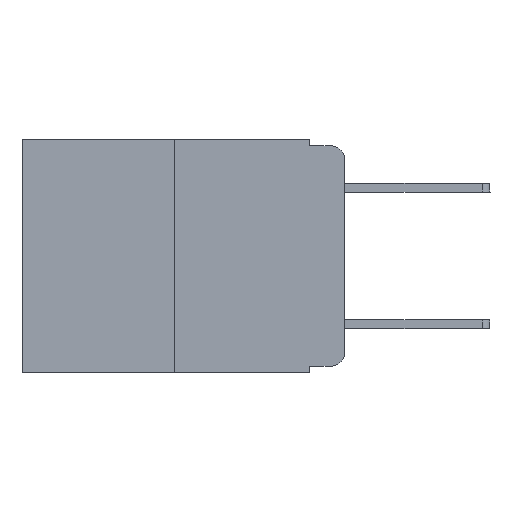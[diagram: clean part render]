
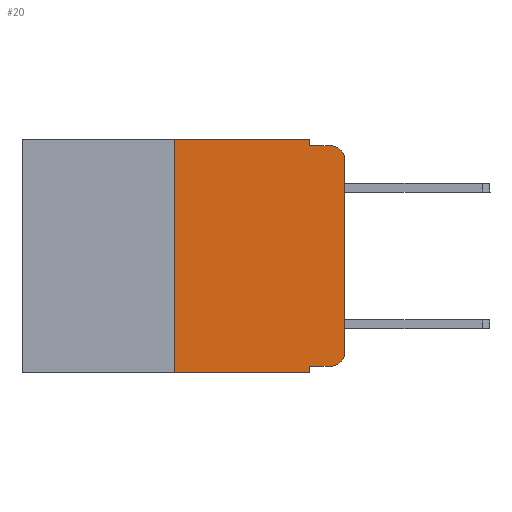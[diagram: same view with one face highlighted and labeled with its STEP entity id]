
A CAD part, left-side view. The second image highlights one B-rep face of the part: STEP entity #20.
In plain terms, the highlighted planar face has unit normal (-1, 0, 0).
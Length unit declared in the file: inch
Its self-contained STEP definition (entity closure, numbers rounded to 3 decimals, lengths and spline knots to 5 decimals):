
#20 = ADVANCED_FACE ( 'NONE', ( #10011 ), #19524, .F. ) ;
#67 = ORIENTED_EDGE ( 'NONE', *, *, #16423, .F. ) ;
#212 = LINE ( 'NONE', #9866, #17922 ) ;
#649 = DIRECTION ( 'NONE',  ( 0., 0., -1. ) ) ;
#1008 = VERTEX_POINT ( 'NONE', #9121 ) ;
#1626 = CIRCLE ( 'NONE', #19811, 0.02 ) ;
#1811 = CARTESIAN_POINT ( 'NONE',  ( 0., 0.051, -0.333 ) ) ;
#1989 = VECTOR ( 'NONE', #13832, 39.37008 ) ;
#2135 = VECTOR ( 'NONE', #3324, 39.37008 ) ;
#2320 = CARTESIAN_POINT ( 'NONE',  ( 0., 0.25, -0.343 ) ) ;
#2354 = EDGE_CURVE ( 'NONE', #8747, #1008, #1626, .T. ) ;
#2454 = VERTEX_POINT ( 'NONE', #3602 ) ;
#2493 = DIRECTION ( 'NONE',  ( 0., -1., 0. ) ) ;
#2894 = DIRECTION ( 'NONE',  ( 0., 0., 1. ) ) ;
#3324 = DIRECTION ( 'NONE',  ( 0., 0., -1. ) ) ;
#3602 = CARTESIAN_POINT ( 'NONE',  ( 0., 0.051, -0.01 ) ) ;
#4012 = EDGE_CURVE ( 'NONE', #2454, #10599, #7758, .T. ) ;
#4350 = CARTESIAN_POINT ( 'NONE',  ( 0., 0.051, -0.01 ) ) ;
#4852 = AXIS2_PLACEMENT_3D ( 'NONE', #17768, #12167, #8105 ) ;
#4875 = CARTESIAN_POINT ( 'NONE',  ( 0., 0., 0. ) ) ;
#5115 = VERTEX_POINT ( 'NONE', #1811 ) ;
#5175 = CARTESIAN_POINT ( 'NONE',  ( 0., 0.25, 0. ) ) ;
#5873 = VECTOR ( 'NONE', #10352, 39.37008 ) ;
#6653 = LINE ( 'NONE', #4875, #22915 ) ;
#7758 = LINE ( 'NONE', #4350, #1989 ) ;
#8105 = DIRECTION ( 'NONE',  ( 0., 0., -1. ) ) ;
#8192 = VECTOR ( 'NONE', #19537, 39.37008 ) ;
#8316 = CARTESIAN_POINT ( 'NONE',  ( 0., 0.051, 0. ) ) ;
#8377 = ORIENTED_EDGE ( 'NONE', *, *, #19294, .T. ) ;
#8747 = VERTEX_POINT ( 'NONE', #16577 ) ;
#8939 = CIRCLE ( 'NONE', #9354, 0.02 ) ;
#9010 = VERTEX_POINT ( 'NONE', #2320 ) ;
#9121 = CARTESIAN_POINT ( 'NONE',  ( 0., 0., -0.313 ) ) ;
#9143 = LINE ( 'NONE', #18397, #2135 ) ;
#9354 = AXIS2_PLACEMENT_3D ( 'NONE', #13157, #12905, #14558 ) ;
#9599 = ORIENTED_EDGE ( 'NONE', *, *, #23957, .T. ) ;
#9866 = CARTESIAN_POINT ( 'NONE',  ( 0., 0.051, -0.333 ) ) ;
#10011 = FACE_OUTER_BOUND ( 'NONE', #17338, .T. ) ;
#10089 = DIRECTION ( 'NONE',  ( 0., -1., 0. ) ) ;
#10352 = DIRECTION ( 'NONE',  ( 0., 0., -1. ) ) ;
#10586 = ORIENTED_EDGE ( 'NONE', *, *, #4012, .F. ) ;
#10599 = VERTEX_POINT ( 'NONE', #20927 ) ;
#10710 = ORIENTED_EDGE ( 'NONE', *, *, #24893, .F. ) ;
#10817 = DIRECTION ( 'NONE',  ( -1., 0., 0. ) ) ;
#12167 = DIRECTION ( 'NONE',  ( 1., 0., 0. ) ) ;
#12524 = ORIENTED_EDGE ( 'NONE', *, *, #22303, .F. ) ;
#12596 = VERTEX_POINT ( 'NONE', #25075 ) ;
#12791 = LINE ( 'NONE', #8316, #5873 ) ;
#12905 = DIRECTION ( 'NONE',  ( -1., 0., 0. ) ) ;
#13157 = CARTESIAN_POINT ( 'NONE',  ( 0., 0.02, -0.03 ) ) ;
#13832 = DIRECTION ( 'NONE',  ( 0., -1., 0. ) ) ;
#14298 = LINE ( 'NONE', #22032, #17835 ) ;
#14558 = DIRECTION ( 'NONE',  ( 0., 0., -1. ) ) ;
#16344 = ORIENTED_EDGE ( 'NONE', *, *, #19044, .T. ) ;
#16423 = EDGE_CURVE ( 'NONE', #16718, #21474, #23723, .T. ) ;
#16533 = EDGE_CURVE ( 'NONE', #5115, #12596, #9143, .T. ) ;
#16577 = CARTESIAN_POINT ( 'NONE',  ( 0., 0.02, -0.333 ) ) ;
#16718 = VERTEX_POINT ( 'NONE', #24993 ) ;
#16779 = VECTOR ( 'NONE', #2894, 39.37008 ) ;
#17338 = EDGE_LOOP ( 'NONE', ( #9599, #8377, #10586, #10710, #67, #12524, #16344, #21961, #19698, #17781 ) ) ;
#17768 = CARTESIAN_POINT ( 'NONE',  ( 0., 0.473, 0. ) ) ;
#17781 = ORIENTED_EDGE ( 'NONE', *, *, #2354, .T. ) ;
#17827 = CARTESIAN_POINT ( 'NONE',  ( 0., 0., -0.03 ) ) ;
#17835 = VECTOR ( 'NONE', #2493, 39.37008 ) ;
#17922 = VECTOR ( 'NONE', #10089, 39.37008 ) ;
#18037 = CARTESIAN_POINT ( 'NONE',  ( 0., 0.02, -0.313 ) ) ;
#18142 = CARTESIAN_POINT ( 'NONE',  ( 0., 0.473, 0. ) ) ;
#18397 = CARTESIAN_POINT ( 'NONE',  ( 0., 0.051, 0. ) ) ;
#19044 = EDGE_CURVE ( 'NONE', #9010, #12596, #14298, .T. ) ;
#19294 = EDGE_CURVE ( 'NONE', #22616, #10599, #8939, .T. ) ;
#19524 = PLANE ( 'NONE',  #4852 ) ;
#19537 = DIRECTION ( 'NONE',  ( 0., -1., 0. ) ) ;
#19698 = ORIENTED_EDGE ( 'NONE', *, *, #20895, .T. ) ;
#19811 = AXIS2_PLACEMENT_3D ( 'NONE', #18037, #10817, #649 ) ;
#20512 = LINE ( 'NONE', #5175, #16779 ) ;
#20895 = EDGE_CURVE ( 'NONE', #5115, #8747, #212, .T. ) ;
#20927 = CARTESIAN_POINT ( 'NONE',  ( 0., 0.02, -0.01 ) ) ;
#21474 = VERTEX_POINT ( 'NONE', #24504 ) ;
#21961 = ORIENTED_EDGE ( 'NONE', *, *, #16533, .F. ) ;
#22032 = CARTESIAN_POINT ( 'NONE',  ( 0., 0.473, -0.343 ) ) ;
#22128 = DIRECTION ( 'NONE',  ( 0., 0., 1. ) ) ;
#22303 = EDGE_CURVE ( 'NONE', #9010, #16718, #20512, .T. ) ;
#22616 = VERTEX_POINT ( 'NONE', #17827 ) ;
#22915 = VECTOR ( 'NONE', #22128, 39.37008 ) ;
#23723 = LINE ( 'NONE', #18142, #8192 ) ;
#23957 = EDGE_CURVE ( 'NONE', #1008, #22616, #6653, .T. ) ;
#24504 = CARTESIAN_POINT ( 'NONE',  ( 0., 0.051, 0. ) ) ;
#24893 = EDGE_CURVE ( 'NONE', #21474, #2454, #12791, .T. ) ;
#24993 = CARTESIAN_POINT ( 'NONE',  ( 0., 0.25, 0. ) ) ;
#25075 = CARTESIAN_POINT ( 'NONE',  ( 0., 0.051, -0.343 ) ) ;
